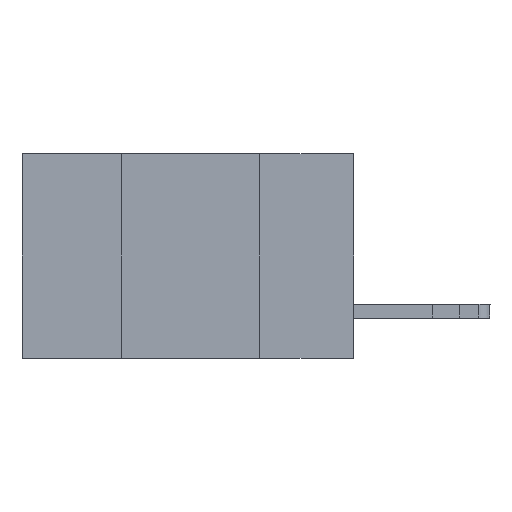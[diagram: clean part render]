
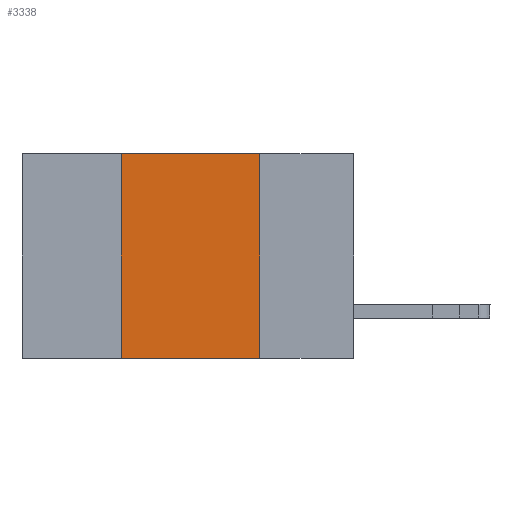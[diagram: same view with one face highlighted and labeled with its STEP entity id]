
A CAD part, left-side view. The second image highlights one B-rep face of the part: STEP entity #3338.
In plain terms, the highlighted planar face has unit normal (-1, 0, 0).
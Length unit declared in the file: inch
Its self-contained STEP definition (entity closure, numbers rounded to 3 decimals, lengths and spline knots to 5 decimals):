
#151 = LINE ( 'NONE', #6670, #5004 ) ;
#826 = DIRECTION ( 'NONE',  ( 0., -1., 0. ) ) ;
#916 = VERTEX_POINT ( 'NONE', #7691 ) ;
#1169 = FACE_OUTER_BOUND ( 'NONE', #9786, .T. ) ;
#1172 = VECTOR ( 'NONE', #4558, 39.37008 ) ;
#1554 = DIRECTION ( 'NONE',  ( 0., 0., -1. ) ) ;
#2505 = DIRECTION ( 'NONE',  ( 1., 0., 0. ) ) ;
#3120 = LINE ( 'NONE', #5790, #1172 ) ;
#3338 = ADVANCED_FACE ( 'NONE', ( #1169 ), #12718, .F. ) ;
#3672 = VERTEX_POINT ( 'NONE', #11759 ) ;
#4084 = CARTESIAN_POINT ( 'NONE',  ( 0., 0.6, 0. ) ) ;
#4558 = DIRECTION ( 'NONE',  ( 0., 0., -1. ) ) ;
#4581 = CARTESIAN_POINT ( 'NONE',  ( 0., 0.42, 0. ) ) ;
#4785 = AXIS2_PLACEMENT_3D ( 'NONE', #7059, #2505, #1554 ) ;
#5004 = VECTOR ( 'NONE', #7722, 39.37008 ) ;
#5102 = EDGE_CURVE ( 'NONE', #916, #12393, #10293, .T. ) ;
#5790 = CARTESIAN_POINT ( 'NONE',  ( 0., 0.17, 0. ) ) ;
#6670 = CARTESIAN_POINT ( 'NONE',  ( 0., 0.6, -0.37 ) ) ;
#6930 = EDGE_CURVE ( 'NONE', #12393, #3672, #7551, .T. ) ;
#7059 = CARTESIAN_POINT ( 'NONE',  ( 0., 0.6, 0. ) ) ;
#7551 = LINE ( 'NONE', #4084, #13703 ) ;
#7691 = CARTESIAN_POINT ( 'NONE',  ( 0., 0.42, -0.37 ) ) ;
#7722 = DIRECTION ( 'NONE',  ( 0., -1., 0. ) ) ;
#8148 = ORIENTED_EDGE ( 'NONE', *, *, #5102, .F. ) ;
#9268 = DIRECTION ( 'NONE',  ( 0., 0., 1. ) ) ;
#9786 = EDGE_LOOP ( 'NONE', ( #13797, #10273, #8148, #12458 ) ) ;
#9931 = VECTOR ( 'NONE', #9268, 39.37008 ) ;
#10273 = ORIENTED_EDGE ( 'NONE', *, *, #6930, .F. ) ;
#10293 = LINE ( 'NONE', #4581, #9931 ) ;
#11759 = CARTESIAN_POINT ( 'NONE',  ( 0., 0.17, 0. ) ) ;
#12393 = VERTEX_POINT ( 'NONE', #12509 ) ;
#12458 = ORIENTED_EDGE ( 'NONE', *, *, #12840, .T. ) ;
#12509 = CARTESIAN_POINT ( 'NONE',  ( 0., 0.42, 0. ) ) ;
#12718 = PLANE ( 'NONE',  #4785 ) ;
#12840 = EDGE_CURVE ( 'NONE', #916, #13989, #151, .T. ) ;
#13103 = CARTESIAN_POINT ( 'NONE',  ( 0., 0.17, -0.37 ) ) ;
#13703 = VECTOR ( 'NONE', #826, 39.37008 ) ;
#13797 = ORIENTED_EDGE ( 'NONE', *, *, #14965, .F. ) ;
#13989 = VERTEX_POINT ( 'NONE', #13103 ) ;
#14965 = EDGE_CURVE ( 'NONE', #3672, #13989, #3120, .T. ) ;
